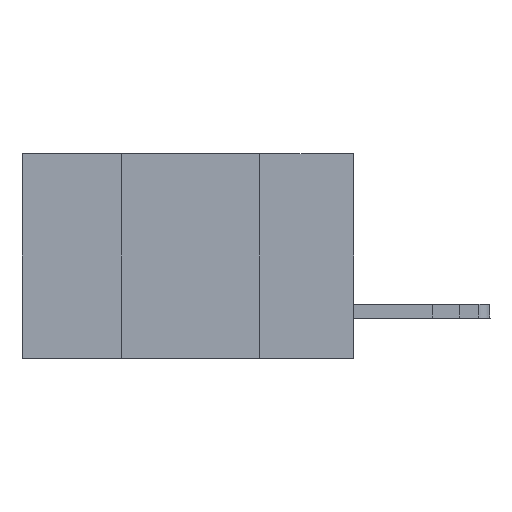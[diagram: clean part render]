
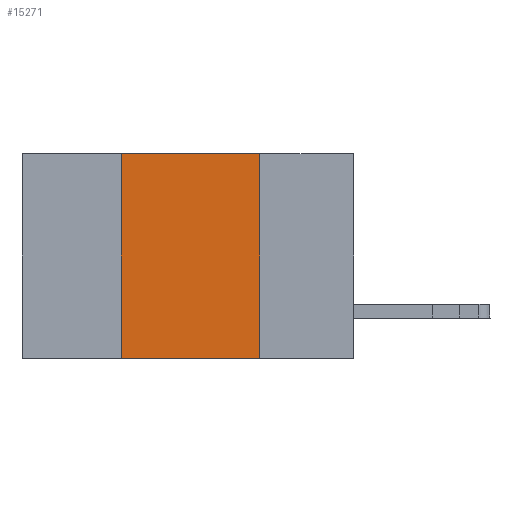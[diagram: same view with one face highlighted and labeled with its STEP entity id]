
A CAD part, left-side view. The second image highlights one B-rep face of the part: STEP entity #15271.
In plain terms, the highlighted planar face has unit normal (-1, 0, 0).
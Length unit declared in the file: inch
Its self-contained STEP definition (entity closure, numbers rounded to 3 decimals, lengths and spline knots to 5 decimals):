
#1043 = VERTEX_POINT ( 'NONE', #7038 ) ;
#1200 = EDGE_CURVE ( 'NONE', #5406, #17384, #14755, .T. ) ;
#1466 = VERTEX_POINT ( 'NONE', #17442 ) ;
#1794 = CARTESIAN_POINT ( 'NONE',  ( 0., 0.42, -0.37 ) ) ;
#2532 = EDGE_CURVE ( 'NONE', #17384, #1043, #19152, .T. ) ;
#3560 = CARTESIAN_POINT ( 'NONE',  ( 0., 0.6, 0. ) ) ;
#4112 = CARTESIAN_POINT ( 'NONE',  ( 0., 0.6, 0. ) ) ;
#5406 = VERTEX_POINT ( 'NONE', #1794 ) ;
#7038 = CARTESIAN_POINT ( 'NONE',  ( 0., 0.17, 0. ) ) ;
#8042 = ORIENTED_EDGE ( 'NONE', *, *, #2532, .F. ) ;
#8912 = EDGE_CURVE ( 'NONE', #5406, #1466, #19549, .T. ) ;
#9227 = VECTOR ( 'NONE', #13618, 39.37008 ) ;
#9728 = CARTESIAN_POINT ( 'NONE',  ( 0., 0.42, 0. ) ) ;
#11277 = AXIS2_PLACEMENT_3D ( 'NONE', #3560, #11580, #11668 ) ;
#11580 = DIRECTION ( 'NONE',  ( 1., 0., 0. ) ) ;
#11668 = DIRECTION ( 'NONE',  ( 0., 0., -1. ) ) ;
#12910 = ORIENTED_EDGE ( 'NONE', *, *, #1200, .F. ) ;
#13141 = DIRECTION ( 'NONE',  ( 0., 0., -1. ) ) ;
#13618 = DIRECTION ( 'NONE',  ( 0., 0., 1. ) ) ;
#13643 = ORIENTED_EDGE ( 'NONE', *, *, #8912, .T. ) ;
#14755 = LINE ( 'NONE', #9728, #9227 ) ;
#15271 = ADVANCED_FACE ( 'NONE', ( #21319 ), #24164, .F. ) ;
#15334 = EDGE_LOOP ( 'NONE', ( #25729, #8042, #12910, #13643 ) ) ;
#16091 = LINE ( 'NONE', #21229, #26381 ) ;
#16199 = DIRECTION ( 'NONE',  ( 0., -1., 0. ) ) ;
#16981 = VECTOR ( 'NONE', #21199, 39.37008 ) ;
#17384 = VERTEX_POINT ( 'NONE', #22291 ) ;
#17442 = CARTESIAN_POINT ( 'NONE',  ( 0., 0.17, -0.37 ) ) ;
#19067 = CARTESIAN_POINT ( 'NONE',  ( 0., 0.6, -0.37 ) ) ;
#19152 = LINE ( 'NONE', #4112, #24612 ) ;
#19549 = LINE ( 'NONE', #19067, #16981 ) ;
#21199 = DIRECTION ( 'NONE',  ( 0., -1., 0. ) ) ;
#21229 = CARTESIAN_POINT ( 'NONE',  ( 0., 0.17, 0. ) ) ;
#21319 = FACE_OUTER_BOUND ( 'NONE', #15334, .T. ) ;
#21635 = EDGE_CURVE ( 'NONE', #1043, #1466, #16091, .T. ) ;
#22291 = CARTESIAN_POINT ( 'NONE',  ( 0., 0.42, 0. ) ) ;
#24164 = PLANE ( 'NONE',  #11277 ) ;
#24612 = VECTOR ( 'NONE', #16199, 39.37008 ) ;
#25729 = ORIENTED_EDGE ( 'NONE', *, *, #21635, .F. ) ;
#26381 = VECTOR ( 'NONE', #13141, 39.37008 ) ;
